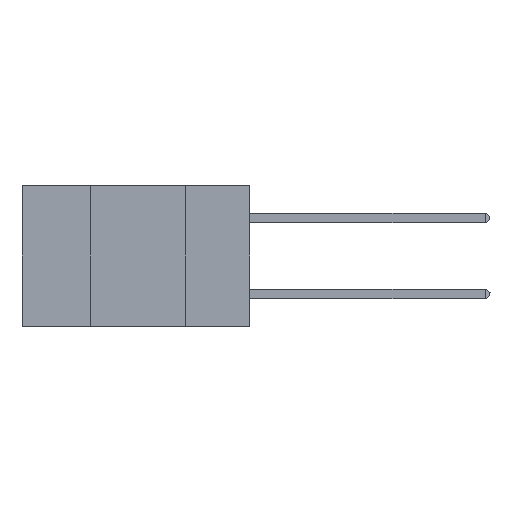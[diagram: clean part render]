
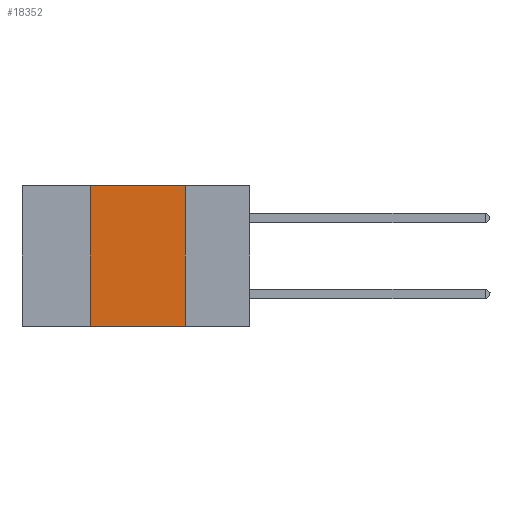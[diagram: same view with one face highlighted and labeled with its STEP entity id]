
A CAD part, left-side view. The second image highlights one B-rep face of the part: STEP entity #18352.
In plain terms, the highlighted planar face has unit normal (-1, 0, 0).
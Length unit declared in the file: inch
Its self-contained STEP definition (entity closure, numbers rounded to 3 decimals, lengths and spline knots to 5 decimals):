
#940 = DIRECTION ( 'NONE',  ( 0., -1., 0. ) ) ;
#2303 = EDGE_CURVE ( 'NONE', #10267, #20478, #28701, .T. ) ;
#3344 = CARTESIAN_POINT ( 'NONE',  ( 0., 0.42, 0. ) ) ;
#4204 = VECTOR ( 'NONE', #41848, 39.37008 ) ;
#5135 = DIRECTION ( 'NONE',  ( 1., 0., 0. ) ) ;
#7616 = VERTEX_POINT ( 'NONE', #22523 ) ;
#8305 = EDGE_CURVE ( 'NONE', #22178, #7616, #41013, .T. ) ;
#8541 = CARTESIAN_POINT ( 'NONE',  ( 0., 0.6, 0. ) ) ;
#9492 = CARTESIAN_POINT ( 'NONE',  ( 0., 0.17, 0. ) ) ;
#10267 = VERTEX_POINT ( 'NONE', #30735 ) ;
#10315 = LINE ( 'NONE', #20030, #33211 ) ;
#12817 = FACE_OUTER_BOUND ( 'NONE', #37660, .T. ) ;
#12849 = LINE ( 'NONE', #37303, #19479 ) ;
#12959 = EDGE_CURVE ( 'NONE', #7616, #10267, #12849, .T. ) ;
#13947 = AXIS2_PLACEMENT_3D ( 'NONE', #8541, #5135, #20982 ) ;
#17829 = DIRECTION ( 'NONE',  ( 0., -1., 0. ) ) ;
#18352 = ADVANCED_FACE ( 'NONE', ( #12817 ), #27650, .F. ) ;
#19479 = VECTOR ( 'NONE', #17829, 39.37008 ) ;
#20030 = CARTESIAN_POINT ( 'NONE',  ( 0., 0.6, -0.37 ) ) ;
#20478 = VERTEX_POINT ( 'NONE', #38452 ) ;
#20982 = DIRECTION ( 'NONE',  ( 0., 0., -1. ) ) ;
#22178 = VERTEX_POINT ( 'NONE', #37749 ) ;
#22523 = CARTESIAN_POINT ( 'NONE',  ( 0., 0.42, 0. ) ) ;
#24145 = EDGE_CURVE ( 'NONE', #22178, #20478, #10315, .T. ) ;
#27650 = PLANE ( 'NONE',  #13947 ) ;
#28369 = ORIENTED_EDGE ( 'NONE', *, *, #2303, .F. ) ;
#28701 = LINE ( 'NONE', #9492, #4204 ) ;
#29227 = ORIENTED_EDGE ( 'NONE', *, *, #12959, .F. ) ;
#29664 = ORIENTED_EDGE ( 'NONE', *, *, #8305, .F. ) ;
#30735 = CARTESIAN_POINT ( 'NONE',  ( 0., 0.17, 0. ) ) ;
#31329 = ORIENTED_EDGE ( 'NONE', *, *, #24145, .T. ) ;
#33211 = VECTOR ( 'NONE', #940, 39.37008 ) ;
#37303 = CARTESIAN_POINT ( 'NONE',  ( 0., 0.6, 0. ) ) ;
#37660 = EDGE_LOOP ( 'NONE', ( #28369, #29227, #29664, #31329 ) ) ;
#37749 = CARTESIAN_POINT ( 'NONE',  ( 0., 0.42, -0.37 ) ) ;
#38452 = CARTESIAN_POINT ( 'NONE',  ( 0., 0.17, -0.37 ) ) ;
#39509 = VECTOR ( 'NONE', #39770, 39.37008 ) ;
#39770 = DIRECTION ( 'NONE',  ( 0., 0., 1. ) ) ;
#41013 = LINE ( 'NONE', #3344, #39509 ) ;
#41848 = DIRECTION ( 'NONE',  ( 0., 0., -1. ) ) ;
